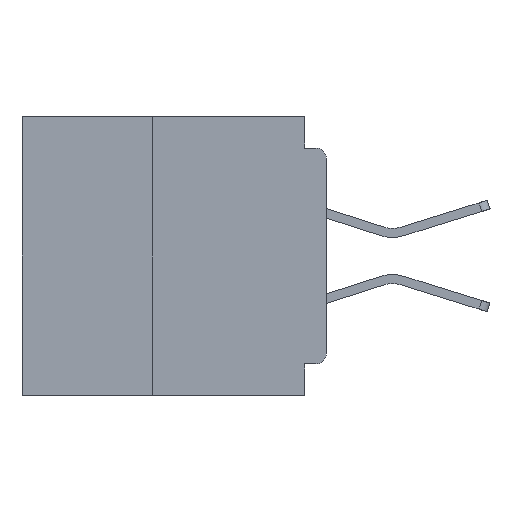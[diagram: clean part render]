
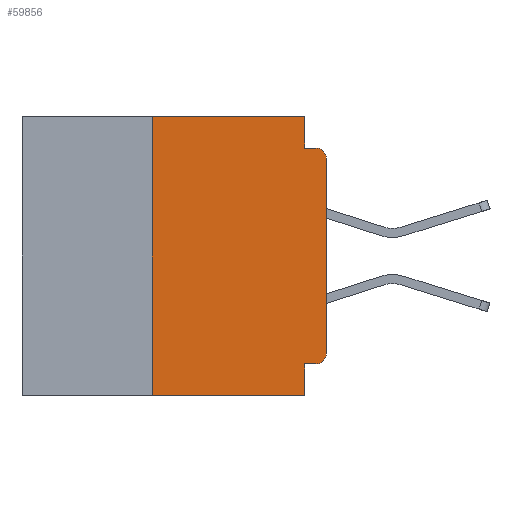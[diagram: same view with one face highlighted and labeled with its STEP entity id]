
A CAD part, left-side view. The second image highlights one B-rep face of the part: STEP entity #59856.
In plain terms, the highlighted planar face has unit normal (-1, 0, 0).
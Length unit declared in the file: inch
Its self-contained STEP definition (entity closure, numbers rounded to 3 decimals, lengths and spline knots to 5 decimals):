
#871 = ORIENTED_EDGE ( 'NONE', *, *, #3520, .F. ) ;
#2149 = CIRCLE ( 'NONE', #49786, 0.015 ) ;
#2298 = PLANE ( 'NONE',  #24772 ) ;
#3520 = EDGE_CURVE ( 'NONE', #42405, #25250, #30270, .T. ) ;
#5660 = CARTESIAN_POINT ( 'NONE',  ( 0., 0.015, -0.06 ) ) ;
#6214 = EDGE_CURVE ( 'NONE', #47270, #25944, #42135, .T. ) ;
#6788 = VERTEX_POINT ( 'NONE', #7511 ) ;
#7192 = VECTOR ( 'NONE', #40502, 39.37008 ) ;
#7511 = CARTESIAN_POINT ( 'NONE',  ( 0., 0.25, -0.4 ) ) ;
#8215 = CARTESIAN_POINT ( 'NONE',  ( 0., 0., -0.34 ) ) ;
#8530 = DIRECTION ( 'NONE',  ( 0., 0., 1. ) ) ;
#9271 = ORIENTED_EDGE ( 'NONE', *, *, #16010, .T. ) ;
#10320 = DIRECTION ( 'NONE',  ( 0., 0., -1. ) ) ;
#10825 = CARTESIAN_POINT ( 'NONE',  ( 0., 0.015, -0.34 ) ) ;
#11054 = DIRECTION ( 'NONE',  ( 0., 0., -1. ) ) ;
#11682 = DIRECTION ( 'NONE',  ( 0., 0., -1. ) ) ;
#12000 = CIRCLE ( 'NONE', #59520, 0.015 ) ;
#12286 = LINE ( 'NONE', #25824, #37066 ) ;
#12787 = EDGE_CURVE ( 'NONE', #55956, #37191, #33598, .T. ) ;
#12903 = EDGE_CURVE ( 'NONE', #6788, #46536, #27787, .T. ) ;
#15500 = DIRECTION ( 'NONE',  ( 0., 0., -1. ) ) ;
#15587 = CARTESIAN_POINT ( 'NONE',  ( 0., 0., -0.045 ) ) ;
#15776 = ORIENTED_EDGE ( 'NONE', *, *, #45682, .F. ) ;
#16010 = EDGE_CURVE ( 'NONE', #6788, #54167, #56491, .T. ) ;
#16931 = CARTESIAN_POINT ( 'NONE',  ( 0., 0.031, -0.355 ) ) ;
#17314 = CARTESIAN_POINT ( 'NONE',  ( 0., 0.437, -0.4 ) ) ;
#17721 = CARTESIAN_POINT ( 'NONE',  ( 0., 0.031, -0.4 ) ) ;
#17778 = VECTOR ( 'NONE', #26415, 39.37008 ) ;
#18915 = VECTOR ( 'NONE', #54573, 39.37008 ) ;
#20272 = DIRECTION ( 'NONE',  ( 0., -1., 0. ) ) ;
#22677 = ORIENTED_EDGE ( 'NONE', *, *, #40511, .T. ) ;
#24772 = AXIS2_PLACEMENT_3D ( 'NONE', #34917, #39550, #11682 ) ;
#24867 = ORIENTED_EDGE ( 'NONE', *, *, #31689, .F. ) ;
#24966 = EDGE_CURVE ( 'NONE', #37191, #53099, #2149, .T. ) ;
#25250 = VERTEX_POINT ( 'NONE', #26420 ) ;
#25824 = CARTESIAN_POINT ( 'NONE',  ( 0., 0.437, 0. ) ) ;
#25944 = VERTEX_POINT ( 'NONE', #16931 ) ;
#26297 = DIRECTION ( 'NONE',  ( 0., 0., 1. ) ) ;
#26324 = VECTOR ( 'NONE', #8530, 39.37008 ) ;
#26415 = DIRECTION ( 'NONE',  ( 0., 0., -1. ) ) ;
#26420 = CARTESIAN_POINT ( 'NONE',  ( 0., 0.031, -0.045 ) ) ;
#26772 = VECTOR ( 'NONE', #11054, 39.37008 ) ;
#27769 = CARTESIAN_POINT ( 'NONE',  ( 0., 0.031, 0. ) ) ;
#27787 = LINE ( 'NONE', #50013, #26324 ) ;
#28394 = ORIENTED_EDGE ( 'NONE', *, *, #12903, .F. ) ;
#30270 = LINE ( 'NONE', #27769, #17778 ) ;
#31689 = EDGE_CURVE ( 'NONE', #25944, #54167, #39103, .T. ) ;
#33598 = LINE ( 'NONE', #53904, #56636 ) ;
#34286 = CARTESIAN_POINT ( 'NONE',  ( 0., 0.031, -0.4 ) ) ;
#34470 = VECTOR ( 'NONE', #20272, 39.37008 ) ;
#34917 = CARTESIAN_POINT ( 'NONE',  ( 0., 0.437, 0. ) ) ;
#36039 = CARTESIAN_POINT ( 'NONE',  ( 0., 0.031, 0. ) ) ;
#36527 = CARTESIAN_POINT ( 'NONE',  ( 0., 0., -0.06 ) ) ;
#36687 = CARTESIAN_POINT ( 'NONE',  ( 0., 0.25, 0. ) ) ;
#37066 = VECTOR ( 'NONE', #53448, 39.37008 ) ;
#37191 = VERTEX_POINT ( 'NONE', #36527 ) ;
#38231 = DIRECTION ( 'NONE',  ( -1., 0., 0. ) ) ;
#38336 = EDGE_LOOP ( 'NONE', ( #52632, #40280, #45521, #871, #15776, #28394, #9271, #24867, #42754, #22677 ) ) ;
#39103 = LINE ( 'NONE', #34286, #26772 ) ;
#39550 = DIRECTION ( 'NONE',  ( 1., 0., 0. ) ) ;
#40280 = ORIENTED_EDGE ( 'NONE', *, *, #24966, .T. ) ;
#40502 = DIRECTION ( 'NONE',  ( 0., -1., 0. ) ) ;
#40511 = EDGE_CURVE ( 'NONE', #47270, #55956, #12000, .T. ) ;
#41636 = EDGE_CURVE ( 'NONE', #25250, #53099, #46678, .T. ) ;
#42135 = LINE ( 'NONE', #45295, #18915 ) ;
#42405 = VERTEX_POINT ( 'NONE', #36039 ) ;
#42754 = ORIENTED_EDGE ( 'NONE', *, *, #6214, .F. ) ;
#43279 = DIRECTION ( 'NONE',  ( -1., 0., 0. ) ) ;
#45009 = CARTESIAN_POINT ( 'NONE',  ( 0., 0.015, -0.045 ) ) ;
#45295 = CARTESIAN_POINT ( 'NONE',  ( 0., 0., -0.355 ) ) ;
#45521 = ORIENTED_EDGE ( 'NONE', *, *, #41636, .F. ) ;
#45682 = EDGE_CURVE ( 'NONE', #46536, #42405, #12286, .T. ) ;
#46536 = VERTEX_POINT ( 'NONE', #36687 ) ;
#46631 = CARTESIAN_POINT ( 'NONE',  ( 0., 0.015, -0.355 ) ) ;
#46678 = LINE ( 'NONE', #15587, #34470 ) ;
#47270 = VERTEX_POINT ( 'NONE', #46631 ) ;
#49786 = AXIS2_PLACEMENT_3D ( 'NONE', #5660, #38231, #10320 ) ;
#50013 = CARTESIAN_POINT ( 'NONE',  ( 0., 0.25, -0.4 ) ) ;
#52632 = ORIENTED_EDGE ( 'NONE', *, *, #12787, .T. ) ;
#53099 = VERTEX_POINT ( 'NONE', #45009 ) ;
#53448 = DIRECTION ( 'NONE',  ( 0., -1., 0. ) ) ;
#53904 = CARTESIAN_POINT ( 'NONE',  ( 0., 0., 0. ) ) ;
#54167 = VERTEX_POINT ( 'NONE', #17721 ) ;
#54573 = DIRECTION ( 'NONE',  ( 0., 1., 0. ) ) ;
#55956 = VERTEX_POINT ( 'NONE', #8215 ) ;
#56491 = LINE ( 'NONE', #17314, #7192 ) ;
#56636 = VECTOR ( 'NONE', #26297, 39.37008 ) ;
#56921 = FACE_OUTER_BOUND ( 'NONE', #38336, .T. ) ;
#59520 = AXIS2_PLACEMENT_3D ( 'NONE', #10825, #43279, #15500 ) ;
#59856 = ADVANCED_FACE ( 'NONE', ( #56921 ), #2298, .F. ) ;
